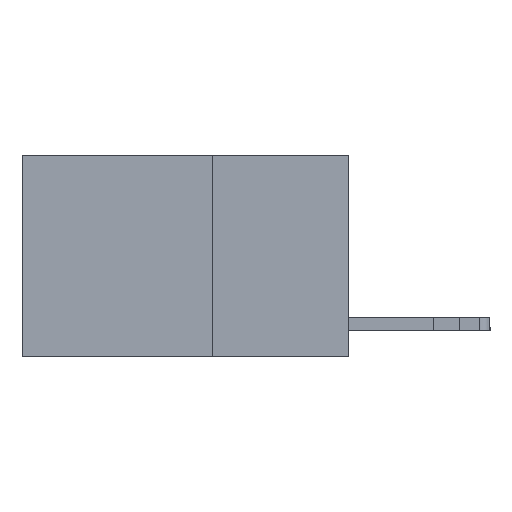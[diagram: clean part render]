
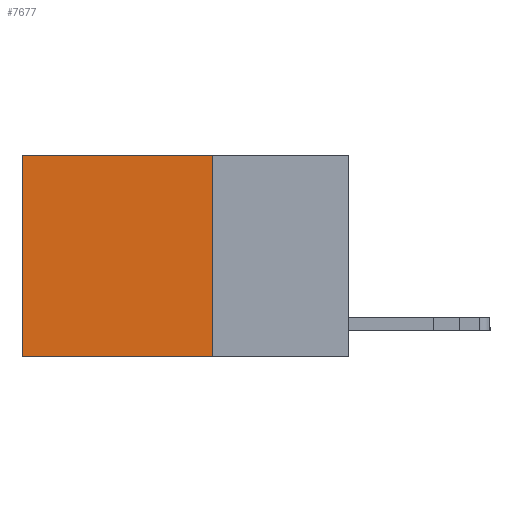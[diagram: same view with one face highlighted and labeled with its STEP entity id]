
A CAD part, left-side view. The second image highlights one B-rep face of the part: STEP entity #7677.
In plain terms, the highlighted planar face has unit normal (-1, 0, 0).
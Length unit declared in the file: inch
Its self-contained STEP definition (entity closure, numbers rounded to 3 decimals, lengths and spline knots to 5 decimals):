
#520 = CARTESIAN_POINT ( 'NONE',  ( 0.2625, 0.6, -0.37 ) ) ;
#656 = EDGE_CURVE ( 'NONE', #4327, #8669, #10394, .T. ) ;
#942 = DIRECTION ( 'NONE',  ( 0., 1., 0. ) ) ;
#1467 = PLANE ( 'NONE',  #5659 ) ;
#1493 = VECTOR ( 'NONE', #5280, 39.37008 ) ;
#1667 = DIRECTION ( 'NONE',  ( 0., 0., -1. ) ) ;
#2176 = VERTEX_POINT ( 'NONE', #6673 ) ;
#2418 = ORIENTED_EDGE ( 'NONE', *, *, #14810, .T. ) ;
#2548 = EDGE_CURVE ( 'NONE', #6873, #2176, #12870, .T. ) ;
#3154 = LINE ( 'NONE', #15177, #3398 ) ;
#3398 = VECTOR ( 'NONE', #1667, 39.37008 ) ;
#3914 = DIRECTION ( 'NONE',  ( 0., 0., -1. ) ) ;
#4327 = VERTEX_POINT ( 'NONE', #15425 ) ;
#5280 = DIRECTION ( 'NONE',  ( 0., 0., -1. ) ) ;
#5659 = AXIS2_PLACEMENT_3D ( 'NONE', #7801, #14899, #3914 ) ;
#6559 = FACE_OUTER_BOUND ( 'NONE', #10554, .T. ) ;
#6673 = CARTESIAN_POINT ( 'NONE',  ( 0.2625, 0.6, 0. ) ) ;
#6681 = CARTESIAN_POINT ( 'NONE',  ( 0.2625, 0.6, 0. ) ) ;
#6873 = VERTEX_POINT ( 'NONE', #12375 ) ;
#7442 = EDGE_CURVE ( 'NONE', #6873, #4327, #3154, .T. ) ;
#7677 = ADVANCED_FACE ( 'NONE', ( #6559 ), #1467, .F. ) ;
#7801 = CARTESIAN_POINT ( 'NONE',  ( 0.2625, 0.25, 0. ) ) ;
#7806 = VECTOR ( 'NONE', #942, 39.37008 ) ;
#8669 = VERTEX_POINT ( 'NONE', #520 ) ;
#8684 = ORIENTED_EDGE ( 'NONE', *, *, #2548, .T. ) ;
#10262 = LINE ( 'NONE', #6681, #1493 ) ;
#10394 = LINE ( 'NONE', #15701, #13283 ) ;
#10554 = EDGE_LOOP ( 'NONE', ( #2418, #16409, #14940, #8684 ) ) ;
#12375 = CARTESIAN_POINT ( 'NONE',  ( 0.2625, 0.25, 0. ) ) ;
#12792 = DIRECTION ( 'NONE',  ( 0., 1., 0. ) ) ;
#12870 = LINE ( 'NONE', #13042, #7806 ) ;
#13042 = CARTESIAN_POINT ( 'NONE',  ( 0.2625, 0.25, 0. ) ) ;
#13283 = VECTOR ( 'NONE', #12792, 39.37008 ) ;
#14810 = EDGE_CURVE ( 'NONE', #2176, #8669, #10262, .T. ) ;
#14899 = DIRECTION ( 'NONE',  ( 1., 0., 0. ) ) ;
#14940 = ORIENTED_EDGE ( 'NONE', *, *, #7442, .F. ) ;
#15177 = CARTESIAN_POINT ( 'NONE',  ( 0.2625, 0.25, 0. ) ) ;
#15425 = CARTESIAN_POINT ( 'NONE',  ( 0.2625, 0.25, -0.37 ) ) ;
#15701 = CARTESIAN_POINT ( 'NONE',  ( 0.2625, 0.25, -0.37 ) ) ;
#16409 = ORIENTED_EDGE ( 'NONE', *, *, #656, .F. ) ;
